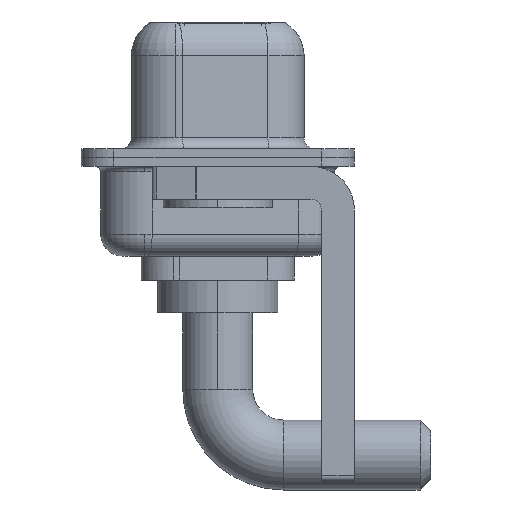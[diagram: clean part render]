
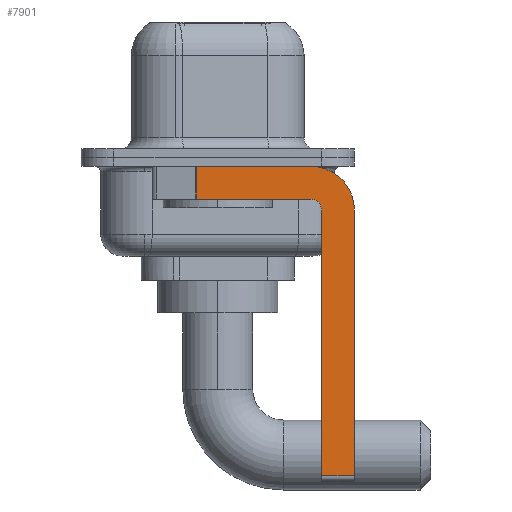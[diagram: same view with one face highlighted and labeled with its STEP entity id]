
A CAD part, left-side view. The second image highlights one B-rep face of the part: STEP entity #7901.
In plain terms, the highlighted planar face has unit normal (-1, 0, 0).
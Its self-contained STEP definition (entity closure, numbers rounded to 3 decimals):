
#46 = DIRECTION ( 'NONE',  ( 0., -1., 0. ) ) ;
#170 = VERTEX_POINT ( 'NONE', #5027 ) ;
#196 = ORIENTED_EDGE ( 'NONE', *, *, #4828, .T. ) ;
#372 = LINE ( 'NONE', #7468, #8168 ) ;
#492 = DIRECTION ( 'NONE',  ( 0., 0., 1. ) ) ;
#557 = DIRECTION ( 'NONE',  ( 0., 0., -1. ) ) ;
#944 = CARTESIAN_POINT ( 'NONE',  ( -2.9, -4.25, -0.4 ) ) ;
#1067 = ORIENTED_EDGE ( 'NONE', *, *, #2562, .T. ) ;
#1090 = ORIENTED_EDGE ( 'NONE', *, *, #5160, .F. ) ;
#1565 = CARTESIAN_POINT ( 'NONE',  ( -2.9, -4.25, -2.4 ) ) ;
#1667 = CARTESIAN_POINT ( 'NONE',  ( -2.9, -4.75, -14.55 ) ) ;
#1783 = DIRECTION ( 'NONE',  ( 0., 0., 1. ) ) ;
#2156 = EDGE_CURVE ( 'NONE', #4163, #170, #7234, .T. ) ;
#2463 = VECTOR ( 'NONE', #46, 1000. ) ;
#2562 = EDGE_CURVE ( 'NONE', #9236, #10552, #3017, .T. ) ;
#2795 = AXIS2_PLACEMENT_3D ( 'NONE', #1565, #11903, #557 ) ;
#3017 = LINE ( 'NONE', #11886, #9568 ) ;
#3044 = DIRECTION ( 'NONE',  ( 0., 0., -1. ) ) ;
#3075 = VECTOR ( 'NONE', #3173, 1000. ) ;
#3173 = DIRECTION ( 'NONE',  ( 0., 1., 0. ) ) ;
#3326 = VECTOR ( 'NONE', #12824, 1000. ) ;
#3507 = AXIS2_PLACEMENT_3D ( 'NONE', #6963, #6762, #1783 ) ;
#3681 = LINE ( 'NONE', #3744, #3326 ) ;
#3744 = CARTESIAN_POINT ( 'NONE',  ( -2.9, 3., -0.4 ) ) ;
#4163 = VERTEX_POINT ( 'NONE', #944 ) ;
#4309 = VERTEX_POINT ( 'NONE', #6442 ) ;
#4445 = VERTEX_POINT ( 'NONE', #1667 ) ;
#4828 = EDGE_CURVE ( 'NONE', #4445, #6108, #9198, .T. ) ;
#5027 = CARTESIAN_POINT ( 'NONE',  ( -2.9, -6.25, -2.4 ) ) ;
#5091 = CARTESIAN_POINT ( 'NONE',  ( -2.9, -4.25, -14.55 ) ) ;
#5149 = CARTESIAN_POINT ( 'NONE',  ( -2.9, -4.25, -1.9 ) ) ;
#5153 = CARTESIAN_POINT ( 'NONE',  ( -2.9, -6.25, -2.4 ) ) ;
#5160 = EDGE_CURVE ( 'NONE', #4309, #10552, #9384, .T. ) ;
#5683 = CARTESIAN_POINT ( 'NONE',  ( -2.9, -4.75, -2.4 ) ) ;
#5685 = DIRECTION ( 'NONE',  ( 1., 0., 0. ) ) ;
#5880 = CARTESIAN_POINT ( 'NONE',  ( -2.9, -6.25, -14.55 ) ) ;
#5889 = VERTEX_POINT ( 'NONE', #5683 ) ;
#6078 = AXIS2_PLACEMENT_3D ( 'NONE', #8125, #5685, #10064 ) ;
#6108 = VERTEX_POINT ( 'NONE', #5880 ) ;
#6442 = CARTESIAN_POINT ( 'NONE',  ( -2.9, -4.25, -1.9 ) ) ;
#6762 = DIRECTION ( 'NONE',  ( -1., 0., 0. ) ) ;
#6963 = CARTESIAN_POINT ( 'NONE',  ( -2.9, -4.25, -2.4 ) ) ;
#7234 = CIRCLE ( 'NONE', #2795, 2. ) ;
#7468 = CARTESIAN_POINT ( 'NONE',  ( -2.9, -4.75, -14.8 ) ) ;
#7699 = ORIENTED_EDGE ( 'NONE', *, *, #2156, .F. ) ;
#7842 = DIRECTION ( 'NONE',  ( 0., 0., -1. ) ) ;
#7901 = ADVANCED_FACE ( 'NONE', ( #12172 ), #9196, .F. ) ;
#7973 = EDGE_CURVE ( 'NONE', #170, #6108, #13038, .T. ) ;
#8125 = CARTESIAN_POINT ( 'NONE',  ( -2.9, -4.25, -2.4 ) ) ;
#8168 = VECTOR ( 'NONE', #492, 1000. ) ;
#8991 = ORIENTED_EDGE ( 'NONE', *, *, #10976, .F. ) ;
#9196 = PLANE ( 'NONE',  #6078 ) ;
#9198 = LINE ( 'NONE', #5091, #2463 ) ;
#9236 = VERTEX_POINT ( 'NONE', #11267 ) ;
#9304 = ORIENTED_EDGE ( 'NONE', *, *, #11692, .F. ) ;
#9351 = ORIENTED_EDGE ( 'NONE', *, *, #7973, .F. ) ;
#9384 = LINE ( 'NONE', #5149, #3075 ) ;
#9477 = VECTOR ( 'NONE', #3044, 1000. ) ;
#9568 = VECTOR ( 'NONE', #7842, 1000. ) ;
#10064 = DIRECTION ( 'NONE',  ( 0., 0., -1. ) ) ;
#10436 = EDGE_LOOP ( 'NONE', ( #12355, #1067, #1090, #8991, #9304, #196, #9351, #7699 ) ) ;
#10552 = VERTEX_POINT ( 'NONE', #11876 ) ;
#10976 = EDGE_CURVE ( 'NONE', #5889, #4309, #13022, .T. ) ;
#11267 = CARTESIAN_POINT ( 'NONE',  ( -2.9, 0.978, -0.4 ) ) ;
#11692 = EDGE_CURVE ( 'NONE', #4445, #5889, #372, .T. ) ;
#11803 = EDGE_CURVE ( 'NONE', #9236, #4163, #3681, .T. ) ;
#11876 = CARTESIAN_POINT ( 'NONE',  ( -2.9, 0.978, -1.9 ) ) ;
#11886 = CARTESIAN_POINT ( 'NONE',  ( -2.9, 0.978, -1.9 ) ) ;
#11903 = DIRECTION ( 'NONE',  ( 1., 0., 0. ) ) ;
#12172 = FACE_OUTER_BOUND ( 'NONE', #10436, .T. ) ;
#12355 = ORIENTED_EDGE ( 'NONE', *, *, #11803, .F. ) ;
#12824 = DIRECTION ( 'NONE',  ( 0., -1., 0. ) ) ;
#13022 = CIRCLE ( 'NONE', #3507, 0.5 ) ;
#13038 = LINE ( 'NONE', #5153, #9477 ) ;
